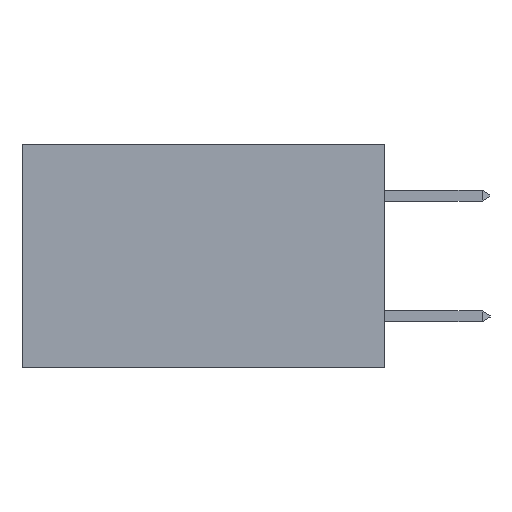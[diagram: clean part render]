
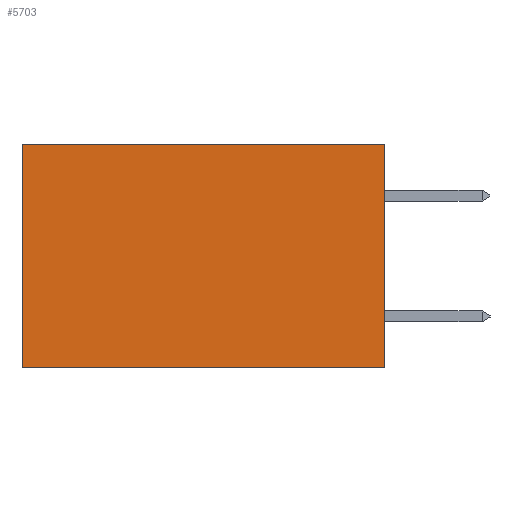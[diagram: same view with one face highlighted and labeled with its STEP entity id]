
A CAD part, left-side view. The second image highlights one B-rep face of the part: STEP entity #5703.
In plain terms, the highlighted planar face has unit normal (-1, 0, 0).
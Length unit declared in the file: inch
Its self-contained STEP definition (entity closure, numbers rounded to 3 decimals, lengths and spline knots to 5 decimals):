
#708 = LINE ( 'NONE', #3057, #26059 ) ;
#2356 = LINE ( 'NONE', #13453, #9124 ) ;
#2387 = VECTOR ( 'NONE', #8375, 39.37008 ) ;
#2697 = VECTOR ( 'NONE', #26367, 39.37008 ) ;
#3057 = CARTESIAN_POINT ( 'NONE',  ( 0.2875, 0.6, 0. ) ) ;
#3297 = CARTESIAN_POINT ( 'NONE',  ( 0.2875, 0.6, -0.37 ) ) ;
#4244 = LINE ( 'NONE', #15347, #2697 ) ;
#5028 = EDGE_CURVE ( 'NONE', #13240, #34286, #4244, .T. ) ;
#5703 = ADVANCED_FACE ( 'NONE', ( #21834 ), #24349, .F. ) ;
#5757 = ORIENTED_EDGE ( 'NONE', *, *, #7137, .F. ) ;
#7137 = EDGE_CURVE ( 'NONE', #34286, #33038, #2356, .T. ) ;
#8375 = DIRECTION ( 'NONE',  ( 0., 1., 0. ) ) ;
#8739 = LINE ( 'NONE', #14038, #2387 ) ;
#9124 = VECTOR ( 'NONE', #21798, 39.37008 ) ;
#10754 = CARTESIAN_POINT ( 'NONE',  ( 0.2875, 0., 0. ) ) ;
#13240 = VERTEX_POINT ( 'NONE', #29496 ) ;
#13453 = CARTESIAN_POINT ( 'NONE',  ( 0.2875, 0., -0.37 ) ) ;
#14038 = CARTESIAN_POINT ( 'NONE',  ( 0.2875, 0., 0. ) ) ;
#15347 = CARTESIAN_POINT ( 'NONE',  ( 0.2875, 0., 0. ) ) ;
#15561 = CARTESIAN_POINT ( 'NONE',  ( 0.2875, 0.6, 0. ) ) ;
#16974 = CARTESIAN_POINT ( 'NONE',  ( 0.2875, 0., -0.37 ) ) ;
#19420 = ORIENTED_EDGE ( 'NONE', *, *, #5028, .F. ) ;
#21629 = VERTEX_POINT ( 'NONE', #15561 ) ;
#21798 = DIRECTION ( 'NONE',  ( 0., 1., 0. ) ) ;
#21834 = FACE_OUTER_BOUND ( 'NONE', #29377, .T. ) ;
#22229 = EDGE_CURVE ( 'NONE', #21629, #33038, #708, .T. ) ;
#23298 = EDGE_CURVE ( 'NONE', #13240, #21629, #8739, .T. ) ;
#24349 = PLANE ( 'NONE',  #35662 ) ;
#26059 = VECTOR ( 'NONE', #28257, 39.37008 ) ;
#26367 = DIRECTION ( 'NONE',  ( 0., 0., -1. ) ) ;
#26768 = ORIENTED_EDGE ( 'NONE', *, *, #22229, .T. ) ;
#28257 = DIRECTION ( 'NONE',  ( 0., 0., -1. ) ) ;
#29377 = EDGE_LOOP ( 'NONE', ( #26768, #5757, #19420, #33351 ) ) ;
#29496 = CARTESIAN_POINT ( 'NONE',  ( 0.2875, 0., 0. ) ) ;
#32674 = DIRECTION ( 'NONE',  ( 0., 0., -1. ) ) ;
#32860 = DIRECTION ( 'NONE',  ( 1., 0., 0. ) ) ;
#33038 = VERTEX_POINT ( 'NONE', #3297 ) ;
#33351 = ORIENTED_EDGE ( 'NONE', *, *, #23298, .T. ) ;
#34286 = VERTEX_POINT ( 'NONE', #16974 ) ;
#35662 = AXIS2_PLACEMENT_3D ( 'NONE', #10754, #32860, #32674 ) ;
